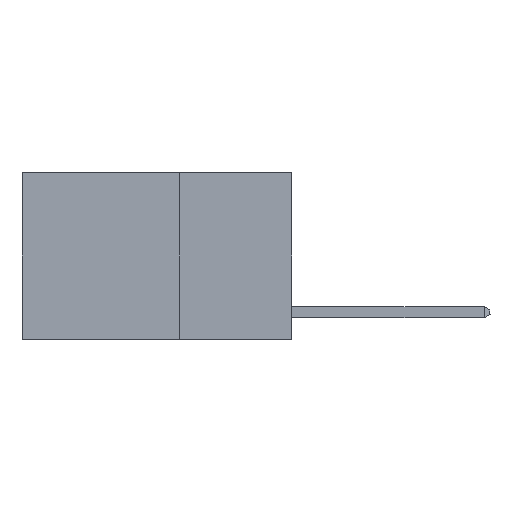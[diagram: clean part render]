
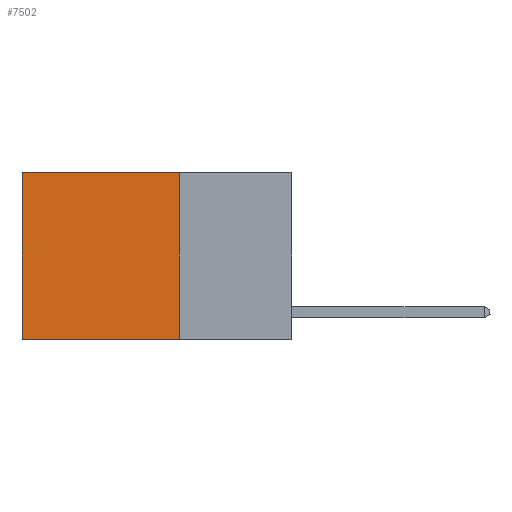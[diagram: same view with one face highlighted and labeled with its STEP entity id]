
A CAD part, left-side view. The second image highlights one B-rep face of the part: STEP entity #7502.
In plain terms, the highlighted planar face has unit normal (-1, 0, 0).
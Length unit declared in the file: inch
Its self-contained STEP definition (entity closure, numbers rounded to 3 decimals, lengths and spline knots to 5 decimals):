
#225 = CARTESIAN_POINT ( 'NONE',  ( 0.2625, 0.25, -0.37 ) ) ;
#822 = VERTEX_POINT ( 'NONE', #4511 ) ;
#956 = EDGE_CURVE ( 'NONE', #16850, #17309, #14335, .T. ) ;
#1496 = ORIENTED_EDGE ( 'NONE', *, *, #14346, .T. ) ;
#2229 = EDGE_CURVE ( 'NONE', #822, #16850, #11908, .T. ) ;
#2820 = ORIENTED_EDGE ( 'NONE', *, *, #10898, .T. ) ;
#2915 = CARTESIAN_POINT ( 'NONE',  ( 0.2625, 0.6, 0. ) ) ;
#3381 = VECTOR ( 'NONE', #7635, 39.37008 ) ;
#3663 = AXIS2_PLACEMENT_3D ( 'NONE', #17493, #5198, #14762 ) ;
#3789 = CARTESIAN_POINT ( 'NONE',  ( 0.2625, 0.25, 0. ) ) ;
#4511 = CARTESIAN_POINT ( 'NONE',  ( 0.2625, 0.25, 0. ) ) ;
#4922 = CARTESIAN_POINT ( 'NONE',  ( 0.2625, 0.25, -0.37 ) ) ;
#5198 = DIRECTION ( 'NONE',  ( 1., 0., 0. ) ) ;
#5768 = EDGE_LOOP ( 'NONE', ( #1496, #6457, #10615, #2820 ) ) ;
#6138 = LINE ( 'NONE', #16963, #13027 ) ;
#6457 = ORIENTED_EDGE ( 'NONE', *, *, #956, .F. ) ;
#6647 = CARTESIAN_POINT ( 'NONE',  ( 0.2625, 0.6, -0.37 ) ) ;
#6660 = CARTESIAN_POINT ( 'NONE',  ( 0.2625, 0.6, 0. ) ) ;
#7358 = LINE ( 'NONE', #6660, #15097 ) ;
#7502 = ADVANCED_FACE ( 'NONE', ( #11856 ), #13413, .F. ) ;
#7635 = DIRECTION ( 'NONE',  ( 0., 1., 0. ) ) ;
#8249 = VECTOR ( 'NONE', #16145, 39.37008 ) ;
#9508 = VERTEX_POINT ( 'NONE', #2915 ) ;
#10615 = ORIENTED_EDGE ( 'NONE', *, *, #2229, .F. ) ;
#10898 = EDGE_CURVE ( 'NONE', #822, #9508, #6138, .T. ) ;
#11856 = FACE_OUTER_BOUND ( 'NONE', #5768, .T. ) ;
#11908 = LINE ( 'NONE', #3789, #8249 ) ;
#13027 = VECTOR ( 'NONE', #15582, 39.37008 ) ;
#13413 = PLANE ( 'NONE',  #3663 ) ;
#14335 = LINE ( 'NONE', #4922, #3381 ) ;
#14346 = EDGE_CURVE ( 'NONE', #9508, #17309, #7358, .T. ) ;
#14762 = DIRECTION ( 'NONE',  ( 0., 0., -1. ) ) ;
#15097 = VECTOR ( 'NONE', #16276, 39.37008 ) ;
#15582 = DIRECTION ( 'NONE',  ( 0., 1., 0. ) ) ;
#16145 = DIRECTION ( 'NONE',  ( 0., 0., -1. ) ) ;
#16276 = DIRECTION ( 'NONE',  ( 0., 0., -1. ) ) ;
#16850 = VERTEX_POINT ( 'NONE', #225 ) ;
#16963 = CARTESIAN_POINT ( 'NONE',  ( 0.2625, 0.25, 0. ) ) ;
#17309 = VERTEX_POINT ( 'NONE', #6647 ) ;
#17493 = CARTESIAN_POINT ( 'NONE',  ( 0.2625, 0.25, 0. ) ) ;
